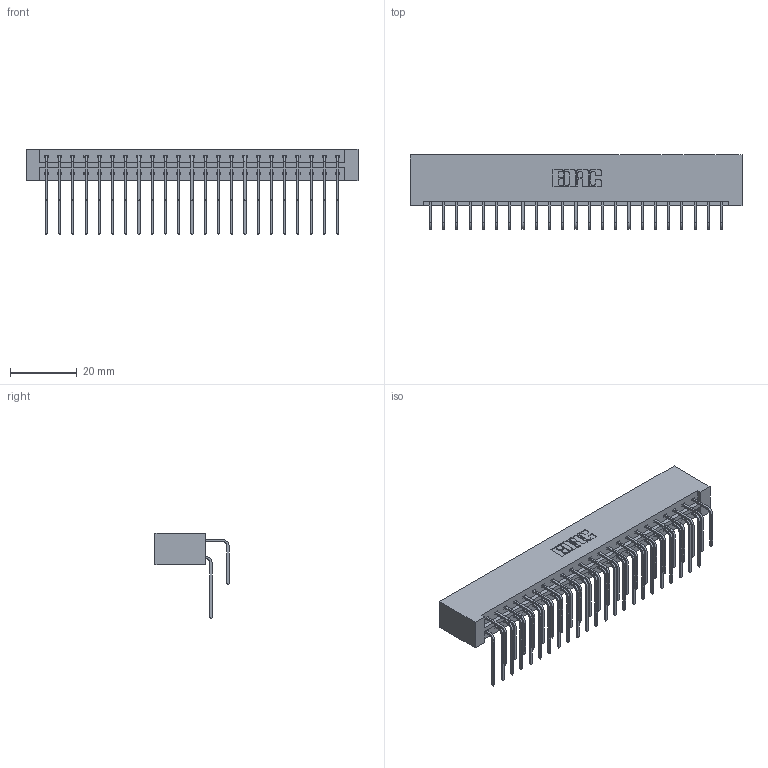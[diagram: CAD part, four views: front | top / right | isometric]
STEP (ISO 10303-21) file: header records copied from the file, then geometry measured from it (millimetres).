
FILE_DESCRIPTION (( 'STEP AP203' ), '1' );
FILE_NAME ('833-046-558-201.STEP', '2020-06-04T14:56:44', ( '' ), ( '' ), 'SwSTEP 2.0', 'SolidWorks 2020', '' );
FILE_SCHEMA (( 'CONFIG_CONTROL_DESIGN' ));
Length unit declared in the file: inch
Products named in the file (4): 833 Part_Lugless; 345-292-001_558 559 Tail - 1; 833-046-558-201; 345-292-001_558 Tail - 2
Assembly tree (47 placements, depth 2):
  833-046-558-201
    833 Part_Lugless
    345-292-001_558 559 Tail - 1  x23
    345-292-001_558 Tail - 2  x23
Bounding box: 99.39 x 22.17 x 25.53 mm (x, y, z)
Volume: 10867.1 mm3; surface area: 13989.6 mm2
Topology: 47 solids, 47 shells, 2590 faces, 7693 edges, 5066 vertices
Faces by surface type: plane 1814, cylinder 776
Entity records: 18761 total; most frequent: CARTESIAN_POINT 3181, ORIENTED_EDGE 3066, DIRECTION 2725, EDGE_CURVE 1533, LINE 1373, VECTOR 1373, VERTEX_POINT 1018, AXIS2_PLACEMENT_3D 676
